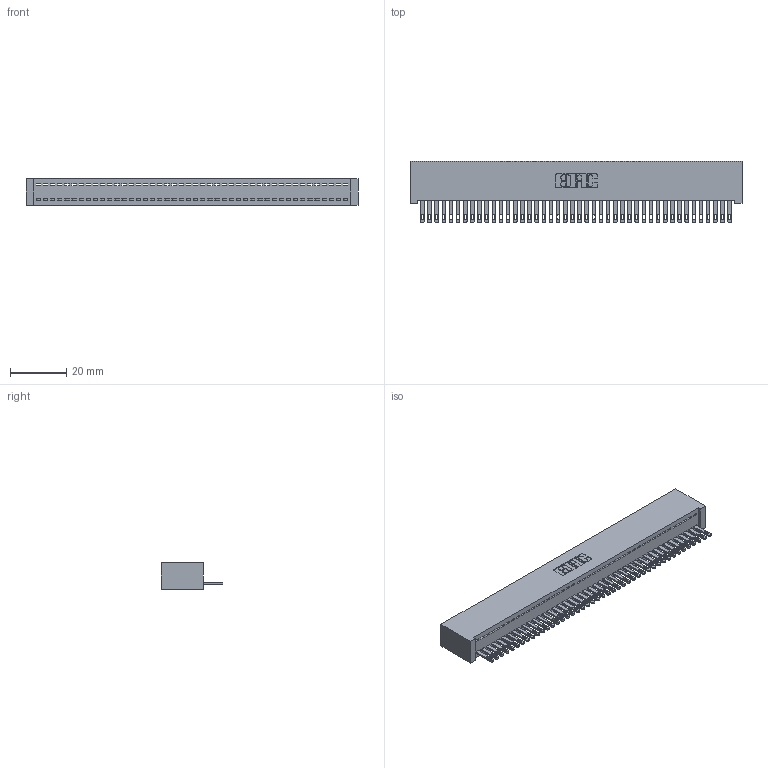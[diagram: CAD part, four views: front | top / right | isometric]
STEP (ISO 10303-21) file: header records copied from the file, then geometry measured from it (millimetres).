
FILE_DESCRIPTION (( 'STEP AP203' ), '1' );
FILE_NAME ('892-044-500-101.STEP', '2020-09-21T16:53:42', ( '' ), ( '' ), 'SwSTEP 2.0', 'SolidWorks 2020', '' );
FILE_SCHEMA (( 'CONFIG_CONTROL_DESIGN' ));
Length unit declared in the file: inch
Products named in the file (3): 345-292-001_345-293-100; 842 Part_Lugless; 892-044-500-101
Assembly tree (45 placements, depth 2):
  892-044-500-101
    842 Part_Lugless
    345-292-001_345-293-100  x44
Bounding box: 118.01 x 21.85 x 9.4 mm (x, y, z)
Volume: 10790.6 mm3; surface area: 16292.7 mm2
Topology: 45 solids, 45 shells, 2478 faces, 7667 edges, 5110 vertices
Faces by surface type: plane 1646, cylinder 832
Entity records: 26161 total; most frequent: CARTESIAN_POINT 4518, ORIENTED_EDGE 4498, DIRECTION 3801, EDGE_CURVE 2249, VECTOR 2125, LINE 2125, VERTEX_POINT 1498, AXIS2_PLACEMENT_3D 838
